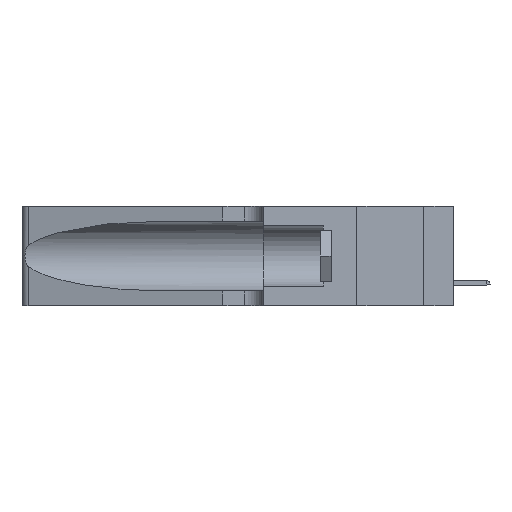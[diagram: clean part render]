
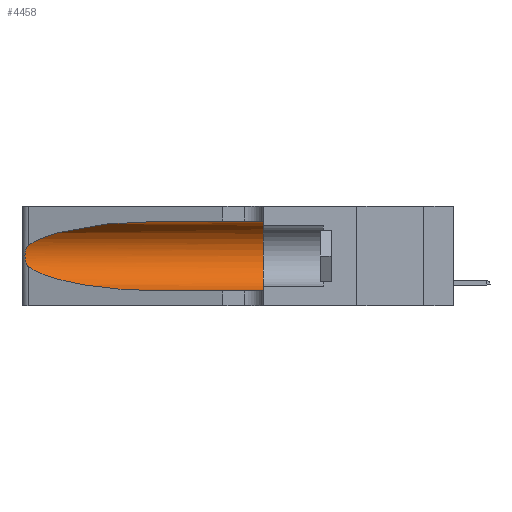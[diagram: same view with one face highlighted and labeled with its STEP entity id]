
A CAD part, left-side view. The second image highlights one B-rep face of the part: STEP entity #4458.
In plain terms, the highlighted cylindrical face has radius 3.308 mm (diameter 6.617 mm), a partial arc.
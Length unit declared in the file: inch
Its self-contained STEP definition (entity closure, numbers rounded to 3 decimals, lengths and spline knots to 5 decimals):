
#440 = CARTESIAN_POINT ( 'NONE',  ( 0.1305, 0.72297, 0.31525 ) ) ;
#667 = AXIS2_PLACEMENT_3D ( 'NONE', #14049, #18654, #10622 ) ;
#1139 = VERTEX_POINT ( 'NONE', #440 ) ;
#1249 = ORIENTED_EDGE ( 'NONE', *, *, #10650, .F. ) ;
#1529 = EDGE_CURVE ( 'NONE', #18255, #8891, #19605, .T. ) ;
#1754 = CARTESIAN_POINT ( 'NONE',  ( 0.1305, 0.72297, 0.05475 ) ) ;
#1806 = CARTESIAN_POINT ( 'NONE',  ( 0.25487, 1.22718, 0.14631 ) ) ;
#2385 = EDGE_CURVE ( 'NONE', #1139, #18255, #17655, .T. ) ;
#2471 = CARTESIAN_POINT ( 'NONE',  ( 0.18966, 0.96281, 0.05475 ) ) ;
#2823 = CARTESIAN_POINT ( 'NONE',  ( 0.26018, 1.23835, 0.19895 ) ) ;
#3536 = CARTESIAN_POINT ( 'NONE',  ( 0.1305, 1.61858, 0.31525 ) ) ;
#3698 = CARTESIAN_POINT ( 'NONE',  ( 0.1305, 0.72297, 0.31525 ) ) ;
#4083 = DIRECTION ( 'NONE',  ( 0., -1., 0. ) ) ;
#4458 = ADVANCED_FACE ( 'NONE', ( #7121 ), #18044, .F. ) ;
#4481 = CARTESIAN_POINT ( 'NONE',  ( 0.1305, 1.61858, 0.05475 ) ) ;
#4928 = VECTOR ( 'NONE', #15946, 39.37008 ) ;
#5569 = DIRECTION ( 'NONE',  ( 0., 0., -1. ) ) ;
#5749 = CARTESIAN_POINT ( 'NONE',  ( 0.25639, 1.23186, 0.15144 ) ) ;
#5939 = CARTESIAN_POINT ( 'NONE',  ( 0.25789, 1.23486, 0.15765 ) ) ;
#6050 = CARTESIAN_POINT ( 'NONE',  ( 0.26075, 1.23896, 0.19203 ) ) ;
#6509 = CARTESIAN_POINT ( 'NONE',  ( 0.18966, 0.96281, 0.31525 ) ) ;
#6781 = VECTOR ( 'NONE', #4083, 39.37008 ) ;
#7121 = FACE_OUTER_BOUND ( 'NONE', #20288, .T. ) ;
#7228 = DIRECTION ( 'NONE',  ( 0., -1., 0. ) ) ;
#8841 = CARTESIAN_POINT ( 'NONE',  ( 0.1305, 0.72297, 0.05475 ) ) ;
#8891 = VERTEX_POINT ( 'NONE', #1806 ) ;
#8903 = CARTESIAN_POINT ( 'NONE',  ( 0.25487, 1.22718, 0.22369 ) ) ;
#9083 = CARTESIAN_POINT ( 'NONE',  ( 0.26075, 1.23896, 0.178 ) ) ;
#9353 =( BOUNDED_CURVE ( )  B_SPLINE_CURVE ( 3, ( #11855, #16665, #2471, #8841 ),
 .UNSPECIFIED., .F., .T. ) 
 B_SPLINE_CURVE_WITH_KNOTS ( ( 4, 4 ),
 ( 3.44316, 4.71239 ),
 .UNSPECIFIED. ) 
 CURVE ( )  GEOMETRIC_REPRESENTATION_ITEM ( )  RATIONAL_B_SPLINE_CURVE ( ( 1., 0.87, 0.87, 1. ) ) 
 REPRESENTATION_ITEM ( '' )  );
#9574 = CIRCLE ( 'NONE', #667, 0.13025 ) ;
#10519 = CARTESIAN_POINT ( 'NONE',  ( 0.25639, 1.23184, 0.21858 ) ) ;
#10622 = DIRECTION ( 'NONE',  ( 0., 0., 1. ) ) ;
#10650 = EDGE_CURVE ( 'NONE', #14414, #11447, #9574, .T. ) ;
#10723 = EDGE_CURVE ( 'NONE', #1139, #14414, #11098, .T. ) ;
#10766 = ORIENTED_EDGE ( 'NONE', *, *, #1529, .T. ) ;
#10859 = VERTEX_POINT ( 'NONE', #1754 ) ;
#11098 = LINE ( 'NONE', #3536, #4928 ) ;
#11447 = VERTEX_POINT ( 'NONE', #19202 ) ;
#11515 = ORIENTED_EDGE ( 'NONE', *, *, #13810, .T. ) ;
#11855 = CARTESIAN_POINT ( 'NONE',  ( 0.25487, 1.22718, 0.14631 ) ) ;
#12005 = CARTESIAN_POINT ( 'NONE',  ( 0.26017, 1.23833, 0.17102 ) ) ;
#12208 = CARTESIAN_POINT ( 'NONE',  ( 0.25555, 1.22994, 0.2215 ) ) ;
#12422 = CARTESIAN_POINT ( 'NONE',  ( 0.25487, 1.22718, 0.14631 ) ) ;
#13436 = CARTESIAN_POINT ( 'NONE',  ( 0.1305, 1.61858, 0.185 ) ) ;
#13521 = CARTESIAN_POINT ( 'NONE',  ( 0.25555, 1.22993, 0.14849 ) ) ;
#13647 = ORIENTED_EDGE ( 'NONE', *, *, #10723, .F. ) ;
#13810 = EDGE_CURVE ( 'NONE', #8891, #10859, #9353, .T. ) ;
#13907 = CARTESIAN_POINT ( 'NONE',  ( 0.1305, 0.35, 0.31525 ) ) ;
#14049 = CARTESIAN_POINT ( 'NONE',  ( 0.1305, 0.35, 0.185 ) ) ;
#14414 = VERTEX_POINT ( 'NONE', #13907 ) ;
#14495 = CARTESIAN_POINT ( 'NONE',  ( 0.2373, 1.15595, 0.28018 ) ) ;
#14702 = CARTESIAN_POINT ( 'NONE',  ( 0.25487, 1.22718, 0.22369 ) ) ;
#15189 = CARTESIAN_POINT ( 'NONE',  ( 0.25856, 1.23593, 0.16098 ) ) ;
#15376 = LINE ( 'NONE', #4481, #6781 ) ;
#15451 = ORIENTED_EDGE ( 'NONE', *, *, #2385, .T. ) ;
#15946 = DIRECTION ( 'NONE',  ( 0., -1., 0. ) ) ;
#16665 = CARTESIAN_POINT ( 'NONE',  ( 0.2373, 1.15595, 0.08982 ) ) ;
#16693 = ORIENTED_EDGE ( 'NONE', *, *, #20286, .T. ) ;
#17655 =( BOUNDED_CURVE ( )  B_SPLINE_CURVE ( 3, ( #3698, #6509, #14495, #14702 ),
 .UNSPECIFIED., .F., .T. ) 
 B_SPLINE_CURVE_WITH_KNOTS ( ( 4, 4 ),
 ( 1.5708, 2.84003 ),
 .UNSPECIFIED. ) 
 CURVE ( )  GEOMETRIC_REPRESENTATION_ITEM ( )  RATIONAL_B_SPLINE_CURVE ( ( 1., 0.87, 0.87, 1. ) ) 
 REPRESENTATION_ITEM ( '' )  );
#17677 = AXIS2_PLACEMENT_3D ( 'NONE', #13436, #7228, #5569 ) ;
#18044 = CYLINDRICAL_SURFACE ( 'NONE', #17677, 0.13025 ) ;
#18255 = VERTEX_POINT ( 'NONE', #18832 ) ;
#18425 = CARTESIAN_POINT ( 'NONE',  ( 0.25787, 1.23484, 0.2124 ) ) ;
#18635 = CARTESIAN_POINT ( 'NONE',  ( 0.25854, 1.2359, 0.20912 ) ) ;
#18654 = DIRECTION ( 'NONE',  ( 0., 1., 0. ) ) ;
#18832 = CARTESIAN_POINT ( 'NONE',  ( 0.25487, 1.22718, 0.22369 ) ) ;
#19202 = CARTESIAN_POINT ( 'NONE',  ( 0.1305, 0.35, 0.05475 ) ) ;
#19605 = B_SPLINE_CURVE_WITH_KNOTS ( 'NONE', 3,
 ( #8903, #12208, #10519, #18425, #18635, #2823, #6050, #9083, #12005, #15189, #5939, #5749, #13521, #12422 ),
 .UNSPECIFIED., .F., .F.,
 ( 4, 2, 2, 2, 2, 2, 4 ),
 ( 0., 0.00027, 0.00053, 0.00107, 0.0016, 0.00187, 0.00214 ),
 .UNSPECIFIED. ) ;
#20286 = EDGE_CURVE ( 'NONE', #10859, #11447, #15376, .T. ) ;
#20288 = EDGE_LOOP ( 'NONE', ( #15451, #10766, #11515, #16693, #1249, #13647 ) ) ;
